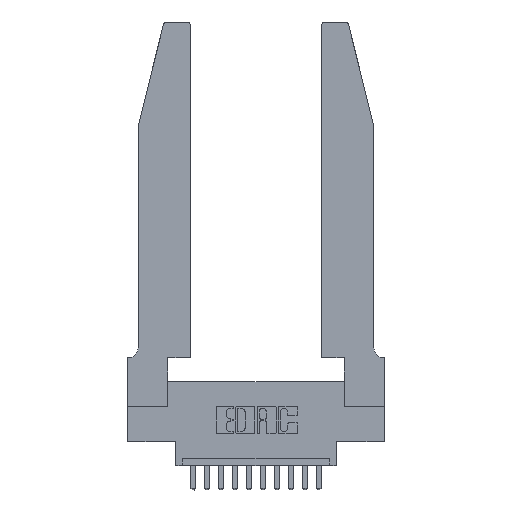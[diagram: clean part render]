
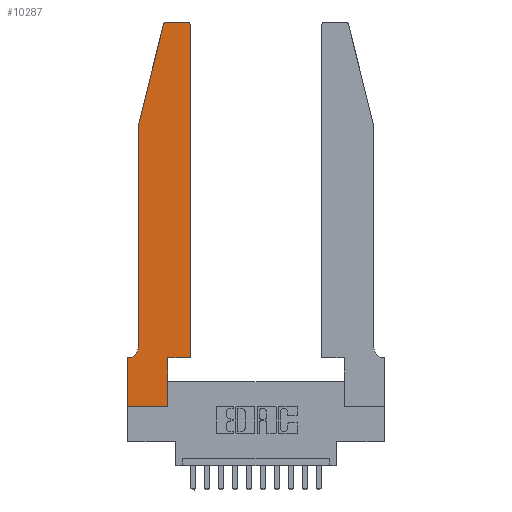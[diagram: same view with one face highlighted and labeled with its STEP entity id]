
A CAD part, top view. The second image highlights one B-rep face of the part: STEP entity #10287.
In plain terms, the highlighted planar face has unit normal (0, 0, 1).
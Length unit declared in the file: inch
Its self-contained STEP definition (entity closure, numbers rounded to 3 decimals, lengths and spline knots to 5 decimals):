
#3 = PLANE ( 'NONE',  #14504 ) ;
#360 = DIRECTION ( 'NONE',  ( -1., 0., 0. ) ) ;
#908 = DIRECTION ( 'NONE',  ( 0., -1., 0. ) ) ;
#1248 = AXIS2_PLACEMENT_3D ( 'NONE', #5909, #5660, #9062 ) ;
#1315 = EDGE_CURVE ( 'NONE', #15331, #10377, #8132, .T. ) ;
#1472 = AXIS2_PLACEMENT_3D ( 'NONE', #6558, #5231, #15591 ) ;
#1492 = ORIENTED_EDGE ( 'NONE', *, *, #1811, .T. ) ;
#1529 = LINE ( 'NONE', #5799, #10478 ) ;
#1805 = EDGE_CURVE ( 'NONE', #8538, #6515, #12337, .T. ) ;
#1811 = EDGE_CURVE ( 'NONE', #8983, #4011, #8753, .T. ) ;
#1831 = VERTEX_POINT ( 'NONE', #3854 ) ;
#1847 = DIRECTION ( 'NONE',  ( -1., 0., 0. ) ) ;
#2305 = CARTESIAN_POINT ( 'NONE',  ( 0., 0., 0.37 ) ) ;
#2349 = EDGE_CURVE ( 'NONE', #10377, #8983, #4426, .T. ) ;
#2382 = CARTESIAN_POINT ( 'NONE',  ( 0.4505, 0.35, 0.37 ) ) ;
#2425 = VECTOR ( 'NONE', #3734, 39.37008 ) ;
#2600 = CARTESIAN_POINT ( 'NONE',  ( 0., 0.35, 0.37 ) ) ;
#2908 = EDGE_CURVE ( 'NONE', #12924, #15331, #13972, .T. ) ;
#2915 = VECTOR ( 'NONE', #15540, 39.37008 ) ;
#3215 = VECTOR ( 'NONE', #11957, 39.37008 ) ;
#3494 = EDGE_CURVE ( 'NONE', #6515, #7281, #1529, .T. ) ;
#3525 = CARTESIAN_POINT ( 'NONE',  ( 0.284, 2.72, 0.37 ) ) ;
#3705 = EDGE_CURVE ( 'NONE', #7281, #9898, #16365, .T. ) ;
#3734 = DIRECTION ( 'NONE',  ( 1., 0., 0. ) ) ;
#3854 = CARTESIAN_POINT ( 'NONE',  ( 0.25487, 2.72718, 0.37 ) ) ;
#4011 = VERTEX_POINT ( 'NONE', #10861 ) ;
#4307 = CARTESIAN_POINT ( 'NONE',  ( 0.4505, 0.35, 0.37 ) ) ;
#4426 = LINE ( 'NONE', #4307, #3215 ) ;
#4487 = ORIENTED_EDGE ( 'NONE', *, *, #1805, .T. ) ;
#4805 = ORIENTED_EDGE ( 'NONE', *, *, #2349, .T. ) ;
#5068 = CARTESIAN_POINT ( 'NONE',  ( 0.2865, 0.35, 0.37 ) ) ;
#5069 = EDGE_CURVE ( 'NONE', #9898, #12924, #15086, .T. ) ;
#5074 = VERTEX_POINT ( 'NONE', #6460 ) ;
#5122 = CARTESIAN_POINT ( 'NONE',  ( 0., 0., 0.37 ) ) ;
#5149 = DIRECTION ( 'NONE',  ( 1., 0., 0. ) ) ;
#5231 = DIRECTION ( 'NONE',  ( 0., 0., 1. ) ) ;
#5456 = EDGE_CURVE ( 'NONE', #5074, #8538, #10806, .T. ) ;
#5531 = CARTESIAN_POINT ( 'NONE',  ( 0.2865, 0.35, 0.37 ) ) ;
#5660 = DIRECTION ( 'NONE',  ( 0., 0., -1. ) ) ;
#5762 = DIRECTION ( 'NONE',  ( 0., -1., 0. ) ) ;
#5799 = CARTESIAN_POINT ( 'NONE',  ( 0.0755, 0.35, 0.37 ) ) ;
#5909 = CARTESIAN_POINT ( 'NONE',  ( 0.0055, 0.42, 0.37 ) ) ;
#6126 = LINE ( 'NONE', #15801, #16219 ) ;
#6460 = CARTESIAN_POINT ( 'NONE',  ( 0.0755, 2., 0.37 ) ) ;
#6515 = VERTEX_POINT ( 'NONE', #14851 ) ;
#6558 = CARTESIAN_POINT ( 'NONE',  ( 0.4205, 2.72, 0.37 ) ) ;
#6757 = ORIENTED_EDGE ( 'NONE', *, *, #16505, .T. ) ;
#6783 = CARTESIAN_POINT ( 'NONE',  ( 0.284, 2.75, 0.37 ) ) ;
#7281 = VERTEX_POINT ( 'NONE', #15820 ) ;
#7542 = FACE_OUTER_BOUND ( 'NONE', #9027, .T. ) ;
#7917 = VECTOR ( 'NONE', #12038, 39.37008 ) ;
#8132 = LINE ( 'NONE', #2382, #2425 ) ;
#8231 = CARTESIAN_POINT ( 'NONE',  ( 0.0755, 2., 0.37 ) ) ;
#8333 = ORIENTED_EDGE ( 'NONE', *, *, #3705, .T. ) ;
#8538 = VERTEX_POINT ( 'NONE', #11256 ) ;
#8753 = CIRCLE ( 'NONE', #1472, 0.03 ) ;
#8983 = VERTEX_POINT ( 'NONE', #10900 ) ;
#9027 = EDGE_LOOP ( 'NONE', ( #6757, #13066, #10395, #15241, #4487, #15461, #8333, #13607, #16293, #10581, #4805, #1492 ) ) ;
#9062 = DIRECTION ( 'NONE',  ( -1., 0., 0. ) ) ;
#9197 = CIRCLE ( 'NONE', #11146, 0.03 ) ;
#9257 = EDGE_CURVE ( 'NONE', #11811, #1831, #9197, .T. ) ;
#9779 = CARTESIAN_POINT ( 'NONE',  ( 0., 0., 0.37 ) ) ;
#9898 = VERTEX_POINT ( 'NONE', #9779 ) ;
#10147 = LINE ( 'NONE', #8231, #7917 ) ;
#10287 = ADVANCED_FACE ( 'NONE', ( #7542 ), #3, .T. ) ;
#10364 = EDGE_CURVE ( 'NONE', #1831, #5074, #10147, .T. ) ;
#10377 = VERTEX_POINT ( 'NONE', #14488 ) ;
#10395 = ORIENTED_EDGE ( 'NONE', *, *, #10364, .T. ) ;
#10478 = VECTOR ( 'NONE', #1847, 39.37008 ) ;
#10581 = ORIENTED_EDGE ( 'NONE', *, *, #1315, .T. ) ;
#10806 = LINE ( 'NONE', #12179, #12833 ) ;
#10861 = CARTESIAN_POINT ( 'NONE',  ( 0.4205, 2.75, 0.37 ) ) ;
#10900 = CARTESIAN_POINT ( 'NONE',  ( 0.4505, 2.72, 0.37 ) ) ;
#11146 = AXIS2_PLACEMENT_3D ( 'NONE', #3525, #13977, #12584 ) ;
#11256 = CARTESIAN_POINT ( 'NONE',  ( 0.0755, 0.42, 0.37 ) ) ;
#11811 = VERTEX_POINT ( 'NONE', #6783 ) ;
#11893 = VECTOR ( 'NONE', #13162, 39.37008 ) ;
#11957 = DIRECTION ( 'NONE',  ( 0., 1., 0. ) ) ;
#12038 = DIRECTION ( 'NONE',  ( -0.239, -0.971, 0. ) ) ;
#12179 = CARTESIAN_POINT ( 'NONE',  ( 0.0755, 2., 0.37 ) ) ;
#12337 = CIRCLE ( 'NONE', #1248, 0.07 ) ;
#12530 = CARTESIAN_POINT ( 'NONE',  ( 0.2865, 0., 0.37 ) ) ;
#12584 = DIRECTION ( 'NONE',  ( 1., 0., 0. ) ) ;
#12833 = VECTOR ( 'NONE', #5762, 39.37008 ) ;
#12903 = DIRECTION ( 'NONE',  ( 0., 0., 1. ) ) ;
#12924 = VERTEX_POINT ( 'NONE', #12530 ) ;
#13066 = ORIENTED_EDGE ( 'NONE', *, *, #9257, .T. ) ;
#13162 = DIRECTION ( 'NONE',  ( 0., 1., 0. ) ) ;
#13607 = ORIENTED_EDGE ( 'NONE', *, *, #5069, .T. ) ;
#13972 = LINE ( 'NONE', #5531, #11893 ) ;
#13977 = DIRECTION ( 'NONE',  ( 0., 0., 1. ) ) ;
#14148 = VECTOR ( 'NONE', #908, 39.37008 ) ;
#14488 = CARTESIAN_POINT ( 'NONE',  ( 0.4505, 0.35, 0.37 ) ) ;
#14504 = AXIS2_PLACEMENT_3D ( 'NONE', #2600, #12903, #5149 ) ;
#14851 = CARTESIAN_POINT ( 'NONE',  ( 0.0055, 0.35, 0.37 ) ) ;
#15086 = LINE ( 'NONE', #5122, #2915 ) ;
#15241 = ORIENTED_EDGE ( 'NONE', *, *, #5456, .T. ) ;
#15331 = VERTEX_POINT ( 'NONE', #5068 ) ;
#15461 = ORIENTED_EDGE ( 'NONE', *, *, #3494, .T. ) ;
#15540 = DIRECTION ( 'NONE',  ( 1., 0., 0. ) ) ;
#15591 = DIRECTION ( 'NONE',  ( 1., 0., 0. ) ) ;
#15801 = CARTESIAN_POINT ( 'NONE',  ( 0.2605, 2.75, 0.37 ) ) ;
#15820 = CARTESIAN_POINT ( 'NONE',  ( 0., 0.35, 0.37 ) ) ;
#16219 = VECTOR ( 'NONE', #360, 39.37008 ) ;
#16293 = ORIENTED_EDGE ( 'NONE', *, *, #2908, .T. ) ;
#16365 = LINE ( 'NONE', #2305, #14148 ) ;
#16505 = EDGE_CURVE ( 'NONE', #4011, #11811, #6126, .T. ) ;
